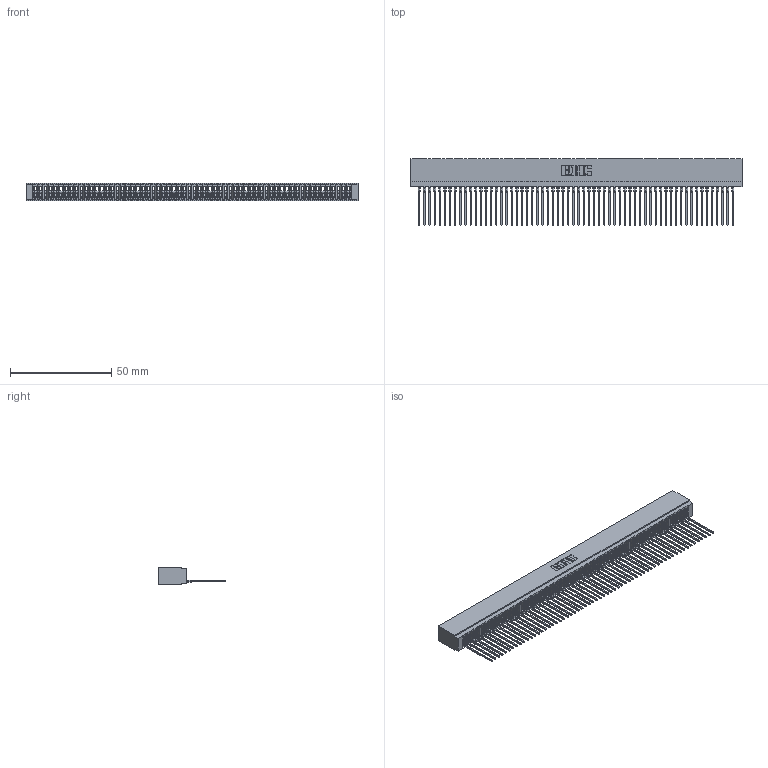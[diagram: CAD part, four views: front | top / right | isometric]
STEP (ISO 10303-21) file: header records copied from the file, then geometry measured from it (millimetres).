
FILE_DESCRIPTION (( 'STEP AP203' ), '1' );
FILE_NAME ('725-062-541-101.STEP', '2026-03-06T00:27:09', ( '' ), ( '' ), 'SwSTEP 2.0', 'SolidWorks 2023', '' );
FILE_SCHEMA (( 'CONFIG_CONTROL_DESIGN' ));
Length unit declared in the file: millimetre
Products named in the file (3): 745-292-001_541; 725-062-541-101; 725 Part_Insulator Option - 01
Assembly tree (63 placements, depth 2):
  725-062-541-101
    725 Part_Insulator Option - 01
    745-292-001_541  x62
Bounding box: 164.08 x 33.03 x 8.89 mm (x, y, z)
Volume: 12607.7 mm3; surface area: 25832 mm2
Topology: 63 solids, 63 shells, 7039 faces, 19350 edges, 12196 vertices
Faces by surface type: plane 4209, bspline 1240, cylinder 1218, torus 372
Entity records: 99628 total; most frequent: CARTESIAN_POINT 18057, ORIENTED_EDGE 17594, DIRECTION 15231, EDGE_CURVE 8797, LINE 8243, VECTOR 8243, VERTEX_POINT 5608, AXIS2_PLACEMENT_3D 3494
